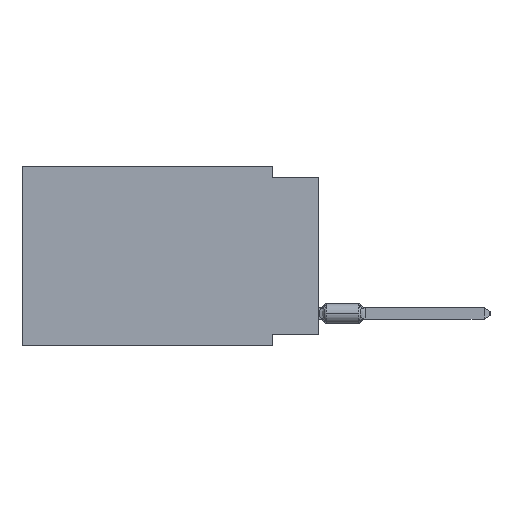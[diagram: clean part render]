
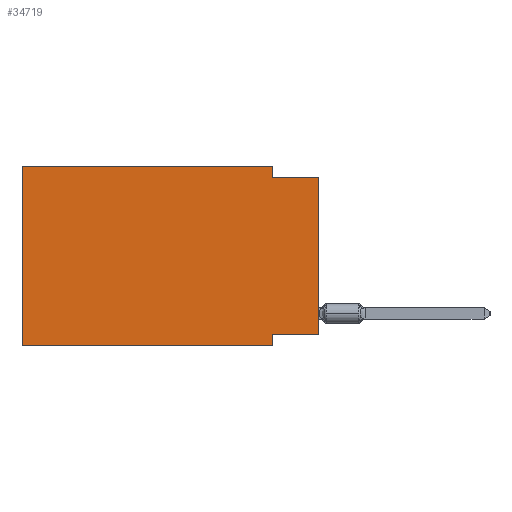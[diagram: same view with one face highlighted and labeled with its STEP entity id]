
A CAD part, left-side view. The second image highlights one B-rep face of the part: STEP entity #34719.
In plain terms, the highlighted planar face has unit normal (-1, 0, 0).
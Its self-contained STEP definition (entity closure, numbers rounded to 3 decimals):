
#38 = DIRECTION ( 'NONE',  ( 0., -1., 0. ) ) ;
#277 = VERTEX_POINT ( 'NONE', #32778 ) ;
#625 = VECTOR ( 'NONE', #11109, 1000. ) ;
#843 = ORIENTED_EDGE ( 'NONE', *, *, #50649, .F. ) ;
#1412 = LINE ( 'NONE', #35395, #71596 ) ;
#3392 = ORIENTED_EDGE ( 'NONE', *, *, #43630, .F. ) ;
#5781 = LINE ( 'NONE', #27012, #75527 ) ;
#5832 = EDGE_CURVE ( 'NONE', #49217, #78582, #25299, .T. ) ;
#7662 = VECTOR ( 'NONE', #57140, 1000. ) ;
#7755 = VECTOR ( 'NONE', #8360, 1000. ) ;
#8109 = DIRECTION ( 'NONE',  ( 0., -1., 0. ) ) ;
#8360 = DIRECTION ( 'NONE',  ( 0., 0., -1. ) ) ;
#9243 = CARTESIAN_POINT ( 'NONE',  ( 0., 2.54, -9.271 ) ) ;
#9570 = EDGE_LOOP ( 'NONE', ( #59008, #56244, #46626, #17907, #3392, #67715, #43390, #843 ) ) ;
#11109 = DIRECTION ( 'NONE',  ( 0., 0., -1. ) ) ;
#17907 = ORIENTED_EDGE ( 'NONE', *, *, #31467, .F. ) ;
#22944 = EDGE_CURVE ( 'NONE', #70216, #29889, #72521, .T. ) ;
#24311 = LINE ( 'NONE', #82484, #625 ) ;
#25299 = LINE ( 'NONE', #56729, #7662 ) ;
#26001 = CARTESIAN_POINT ( 'NONE',  ( 0., 16.383, 0. ) ) ;
#27012 = CARTESIAN_POINT ( 'NONE',  ( 0., 16.383, 0. ) ) ;
#27787 = VECTOR ( 'NONE', #34223, 1000. ) ;
#28166 = CARTESIAN_POINT ( 'NONE',  ( 0., 2.54, -9.906 ) ) ;
#28899 = VECTOR ( 'NONE', #8109, 1000. ) ;
#29889 = VERTEX_POINT ( 'NONE', #28166 ) ;
#31467 = EDGE_CURVE ( 'NONE', #277, #37586, #51492, .T. ) ;
#32778 = CARTESIAN_POINT ( 'NONE',  ( 0., 16.383, 0. ) ) ;
#33909 = PLANE ( 'NONE',  #53696 ) ;
#34223 = DIRECTION ( 'NONE',  ( 0., -1., 0. ) ) ;
#34719 = ADVANCED_FACE ( 'NONE', ( #64611 ), #33909, .F. ) ;
#35395 = CARTESIAN_POINT ( 'NONE',  ( 0., 0., -9.271 ) ) ;
#36178 = VERTEX_POINT ( 'NONE', #81949 ) ;
#37586 = VERTEX_POINT ( 'NONE', #41127 ) ;
#38252 = CARTESIAN_POINT ( 'NONE',  ( 0., 0., -9.271 ) ) ;
#40878 = CARTESIAN_POINT ( 'NONE',  ( 0., 2.54, -0.635 ) ) ;
#41127 = CARTESIAN_POINT ( 'NONE',  ( 0., 2.54, 0. ) ) ;
#43390 = ORIENTED_EDGE ( 'NONE', *, *, #22944, .F. ) ;
#43630 = EDGE_CURVE ( 'NONE', #36178, #277, #5781, .T. ) ;
#44668 = CARTESIAN_POINT ( 'NONE',  ( 0., 16.383, 0. ) ) ;
#46626 = ORIENTED_EDGE ( 'NONE', *, *, #60387, .F. ) ;
#46648 = VERTEX_POINT ( 'NONE', #40878 ) ;
#46888 = DIRECTION ( 'NONE',  ( 0., 1., 0. ) ) ;
#49217 = VERTEX_POINT ( 'NONE', #38252 ) ;
#50521 = CARTESIAN_POINT ( 'NONE',  ( 0., 0., -0.635 ) ) ;
#50649 = EDGE_CURVE ( 'NONE', #49217, #70216, #1412, .T. ) ;
#51492 = LINE ( 'NONE', #26001, #28899 ) ;
#52516 = LINE ( 'NONE', #71616, #27787 ) ;
#53696 = AXIS2_PLACEMENT_3D ( 'NONE', #44668, #66180, #64185 ) ;
#56244 = ORIENTED_EDGE ( 'NONE', *, *, #60566, .F. ) ;
#56729 = CARTESIAN_POINT ( 'NONE',  ( 0., 0., 0. ) ) ;
#57140 = DIRECTION ( 'NONE',  ( 0., 0., 1. ) ) ;
#59008 = ORIENTED_EDGE ( 'NONE', *, *, #5832, .T. ) ;
#59373 = CARTESIAN_POINT ( 'NONE',  ( 0., 2.54, -9.906 ) ) ;
#60387 = EDGE_CURVE ( 'NONE', #37586, #46648, #24311, .T. ) ;
#60566 = EDGE_CURVE ( 'NONE', #46648, #78582, #72232, .T. ) ;
#64185 = DIRECTION ( 'NONE',  ( 0., 0., -1. ) ) ;
#64611 = FACE_OUTER_BOUND ( 'NONE', #9570, .T. ) ;
#66180 = DIRECTION ( 'NONE',  ( 1., 0., 0. ) ) ;
#67715 = ORIENTED_EDGE ( 'NONE', *, *, #84027, .T. ) ;
#70216 = VERTEX_POINT ( 'NONE', #9243 ) ;
#70767 = DIRECTION ( 'NONE',  ( 0., 0., 1. ) ) ;
#71596 = VECTOR ( 'NONE', #46888, 1000. ) ;
#71616 = CARTESIAN_POINT ( 'NONE',  ( 0., 16.383, -9.906 ) ) ;
#72232 = LINE ( 'NONE', #78187, #72553 ) ;
#72521 = LINE ( 'NONE', #59373, #7755 ) ;
#72553 = VECTOR ( 'NONE', #38, 1000. ) ;
#75527 = VECTOR ( 'NONE', #70767, 1000. ) ;
#78187 = CARTESIAN_POINT ( 'NONE',  ( 0., 0., -0.635 ) ) ;
#78582 = VERTEX_POINT ( 'NONE', #50521 ) ;
#81949 = CARTESIAN_POINT ( 'NONE',  ( 0., 16.383, -9.906 ) ) ;
#82484 = CARTESIAN_POINT ( 'NONE',  ( 0., 2.54, 0. ) ) ;
#84027 = EDGE_CURVE ( 'NONE', #36178, #29889, #52516, .T. ) ;
